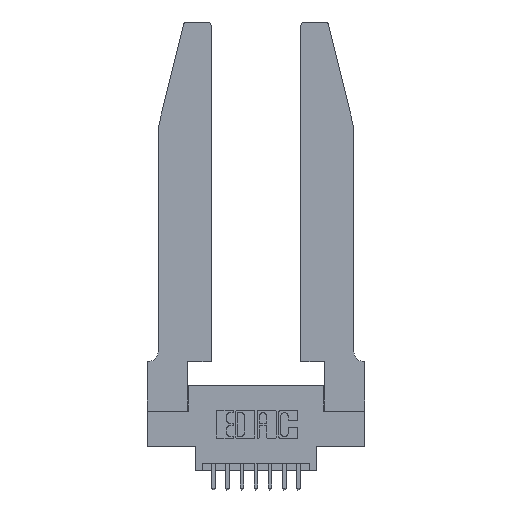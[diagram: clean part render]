
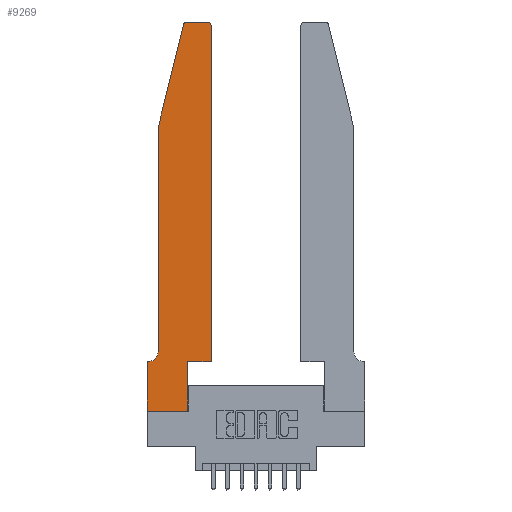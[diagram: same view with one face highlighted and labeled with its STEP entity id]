
A CAD part, top view. The second image highlights one B-rep face of the part: STEP entity #9269.
In plain terms, the highlighted planar face has unit normal (0, 0, 1).
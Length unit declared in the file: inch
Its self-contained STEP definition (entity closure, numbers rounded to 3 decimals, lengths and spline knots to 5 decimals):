
#263 = VERTEX_POINT ( 'NONE', #10458 ) ;
#298 = VERTEX_POINT ( 'NONE', #8187 ) ;
#401 = EDGE_CURVE ( 'NONE', #298, #263, #5202, .T. ) ;
#781 = DIRECTION ( 'NONE',  ( -1., 0., 0. ) ) ;
#811 = DIRECTION ( 'NONE',  ( 0., 1., 0. ) ) ;
#852 = CARTESIAN_POINT ( 'NONE',  ( 0.2865, 0.35, 0.37 ) ) ;
#959 = CARTESIAN_POINT ( 'NONE',  ( 0.0055, 0.35, 0.37 ) ) ;
#1154 = CIRCLE ( 'NONE', #9030, 0.03 ) ;
#1232 = DIRECTION ( 'NONE',  ( 1., 0., 0. ) ) ;
#1260 = LINE ( 'NONE', #14627, #8551 ) ;
#1296 = FACE_OUTER_BOUND ( 'NONE', #4113, .T. ) ;
#1469 = LINE ( 'NONE', #15109, #9645 ) ;
#1493 = CARTESIAN_POINT ( 'NONE',  ( 0.0755, 0.35, 0.37 ) ) ;
#1541 = CARTESIAN_POINT ( 'NONE',  ( 0.4205, 2.75, 0.37 ) ) ;
#1542 = CARTESIAN_POINT ( 'NONE',  ( 0., 0., 0.37 ) ) ;
#1812 = VERTEX_POINT ( 'NONE', #8658 ) ;
#1894 = ORIENTED_EDGE ( 'NONE', *, *, #3141, .T. ) ;
#2319 = VECTOR ( 'NONE', #6101, 39.37008 ) ;
#2462 = LINE ( 'NONE', #2799, #14529 ) ;
#2574 = CIRCLE ( 'NONE', #3224, 0.07 ) ;
#2584 = DIRECTION ( 'NONE',  ( 0., -1., 0. ) ) ;
#2698 = CARTESIAN_POINT ( 'NONE',  ( 0.0755, 2., 0.37 ) ) ;
#2799 = CARTESIAN_POINT ( 'NONE',  ( 0.4505, 0.35, 0.37 ) ) ;
#3027 = CARTESIAN_POINT ( 'NONE',  ( 0.4505, 0.35, 0.37 ) ) ;
#3040 = CARTESIAN_POINT ( 'NONE',  ( 0.284, 2.75, 0.37 ) ) ;
#3057 = CARTESIAN_POINT ( 'NONE',  ( 0.0055, 0.42, 0.37 ) ) ;
#3076 = DIRECTION ( 'NONE',  ( 0., 0., 1. ) ) ;
#3141 = EDGE_CURVE ( 'NONE', #3726, #3333, #4228, .T. ) ;
#3224 = AXIS2_PLACEMENT_3D ( 'NONE', #3057, #6533, #781 ) ;
#3303 = DIRECTION ( 'NONE',  ( 0., -1., 0. ) ) ;
#3316 = EDGE_CURVE ( 'NONE', #263, #13725, #2574, .T. ) ;
#3333 = VERTEX_POINT ( 'NONE', #9050 ) ;
#3461 = EDGE_CURVE ( 'NONE', #10012, #298, #1469, .T. ) ;
#3464 = VERTEX_POINT ( 'NONE', #5622 ) ;
#3500 = DIRECTION ( 'NONE',  ( -0.239, -0.971, 0. ) ) ;
#3571 = LINE ( 'NONE', #1493, #2319 ) ;
#3726 = VERTEX_POINT ( 'NONE', #852 ) ;
#3809 = DIRECTION ( 'NONE',  ( 1., 0., 0. ) ) ;
#4113 = EDGE_LOOP ( 'NONE', ( #9351, #13807, #14636, #12008, #14938, #14747, #6170, #10098, #10675, #1894, #6013, #7431 ) ) ;
#4228 = LINE ( 'NONE', #3027, #10578 ) ;
#4449 = EDGE_CURVE ( 'NONE', #5457, #5710, #1260, .T. ) ;
#4665 = VERTEX_POINT ( 'NONE', #10255 ) ;
#4721 = AXIS2_PLACEMENT_3D ( 'NONE', #11856, #10727, #3809 ) ;
#4837 = DIRECTION ( 'NONE',  ( 0., 0., 1. ) ) ;
#5056 = LINE ( 'NONE', #1542, #10858 ) ;
#5202 = LINE ( 'NONE', #2698, #12287 ) ;
#5457 = VERTEX_POINT ( 'NONE', #1541 ) ;
#5593 = DIRECTION ( 'NONE',  ( 1., 0., 0. ) ) ;
#5622 = CARTESIAN_POINT ( 'NONE',  ( 0., 0.35, 0.37 ) ) ;
#5623 = LINE ( 'NONE', #5846, #6353 ) ;
#5710 = VERTEX_POINT ( 'NONE', #3040 ) ;
#5846 = CARTESIAN_POINT ( 'NONE',  ( 0.2865, 0.35, 0.37 ) ) ;
#5938 = EDGE_CURVE ( 'NONE', #14058, #3726, #5623, .T. ) ;
#6013 = ORIENTED_EDGE ( 'NONE', *, *, #7742, .T. ) ;
#6033 = PLANE ( 'NONE',  #4721 ) ;
#6101 = DIRECTION ( 'NONE',  ( -1., 0., 0. ) ) ;
#6109 = EDGE_CURVE ( 'NONE', #3464, #1812, #13441, .T. ) ;
#6170 = ORIENTED_EDGE ( 'NONE', *, *, #6109, .T. ) ;
#6317 = DIRECTION ( 'NONE',  ( 1., 0., 0. ) ) ;
#6353 = VECTOR ( 'NONE', #811, 39.37008 ) ;
#6533 = DIRECTION ( 'NONE',  ( 0., 0., -1. ) ) ;
#6628 = AXIS2_PLACEMENT_3D ( 'NONE', #10577, #4837, #1232 ) ;
#6707 = EDGE_CURVE ( 'NONE', #1812, #14058, #5056, .T. ) ;
#6768 = EDGE_CURVE ( 'NONE', #13725, #3464, #3571, .T. ) ;
#7246 = VECTOR ( 'NONE', #3303, 39.37008 ) ;
#7431 = ORIENTED_EDGE ( 'NONE', *, *, #10518, .T. ) ;
#7742 = EDGE_CURVE ( 'NONE', #3333, #4665, #2462, .T. ) ;
#7772 = CARTESIAN_POINT ( 'NONE',  ( 0.284, 2.72, 0.37 ) ) ;
#8187 = CARTESIAN_POINT ( 'NONE',  ( 0.0755, 2., 0.37 ) ) ;
#8551 = VECTOR ( 'NONE', #12299, 39.37008 ) ;
#8658 = CARTESIAN_POINT ( 'NONE',  ( 0., 0., 0.37 ) ) ;
#9030 = AXIS2_PLACEMENT_3D ( 'NONE', #7772, #3076, #5593 ) ;
#9050 = CARTESIAN_POINT ( 'NONE',  ( 0.4505, 0.35, 0.37 ) ) ;
#9269 = ADVANCED_FACE ( 'NONE', ( #1296 ), #6033, .T. ) ;
#9351 = ORIENTED_EDGE ( 'NONE', *, *, #4449, .T. ) ;
#9645 = VECTOR ( 'NONE', #3500, 39.37008 ) ;
#10012 = VERTEX_POINT ( 'NONE', #12027 ) ;
#10098 = ORIENTED_EDGE ( 'NONE', *, *, #6707, .T. ) ;
#10192 = EDGE_CURVE ( 'NONE', #5710, #10012, #1154, .T. ) ;
#10255 = CARTESIAN_POINT ( 'NONE',  ( 0.4505, 2.72, 0.37 ) ) ;
#10458 = CARTESIAN_POINT ( 'NONE',  ( 0.0755, 0.42, 0.37 ) ) ;
#10518 = EDGE_CURVE ( 'NONE', #4665, #5457, #13905, .T. ) ;
#10577 = CARTESIAN_POINT ( 'NONE',  ( 0.4205, 2.72, 0.37 ) ) ;
#10578 = VECTOR ( 'NONE', #14707, 39.37008 ) ;
#10675 = ORIENTED_EDGE ( 'NONE', *, *, #5938, .T. ) ;
#10727 = DIRECTION ( 'NONE',  ( 0., 0., 1. ) ) ;
#10858 = VECTOR ( 'NONE', #6317, 39.37008 ) ;
#11856 = CARTESIAN_POINT ( 'NONE',  ( 0., 0.35, 0.37 ) ) ;
#12008 = ORIENTED_EDGE ( 'NONE', *, *, #401, .T. ) ;
#12027 = CARTESIAN_POINT ( 'NONE',  ( 0.25487, 2.72718, 0.37 ) ) ;
#12287 = VECTOR ( 'NONE', #2584, 39.37008 ) ;
#12299 = DIRECTION ( 'NONE',  ( -1., 0., 0. ) ) ;
#12362 = CARTESIAN_POINT ( 'NONE',  ( 0., 0., 0.37 ) ) ;
#13289 = DIRECTION ( 'NONE',  ( 0., 1., 0. ) ) ;
#13441 = LINE ( 'NONE', #12362, #7246 ) ;
#13725 = VERTEX_POINT ( 'NONE', #959 ) ;
#13807 = ORIENTED_EDGE ( 'NONE', *, *, #10192, .T. ) ;
#13905 = CIRCLE ( 'NONE', #6628, 0.03 ) ;
#14058 = VERTEX_POINT ( 'NONE', #14458 ) ;
#14458 = CARTESIAN_POINT ( 'NONE',  ( 0.2865, 0., 0.37 ) ) ;
#14529 = VECTOR ( 'NONE', #13289, 39.37008 ) ;
#14627 = CARTESIAN_POINT ( 'NONE',  ( 0.2605, 2.75, 0.37 ) ) ;
#14636 = ORIENTED_EDGE ( 'NONE', *, *, #3461, .T. ) ;
#14707 = DIRECTION ( 'NONE',  ( 1., 0., 0. ) ) ;
#14747 = ORIENTED_EDGE ( 'NONE', *, *, #6768, .T. ) ;
#14938 = ORIENTED_EDGE ( 'NONE', *, *, #3316, .T. ) ;
#15109 = CARTESIAN_POINT ( 'NONE',  ( 0.0755, 2., 0.37 ) ) ;
